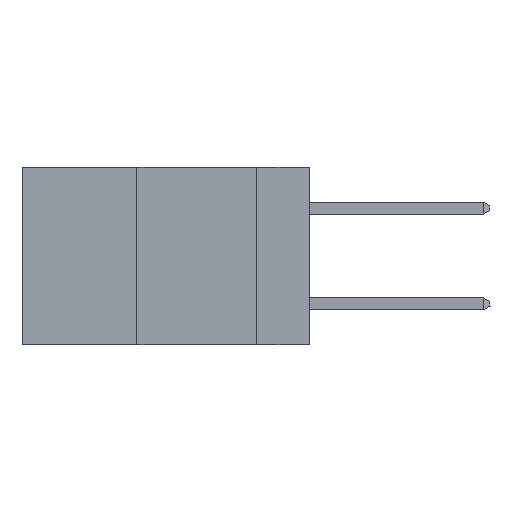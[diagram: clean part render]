
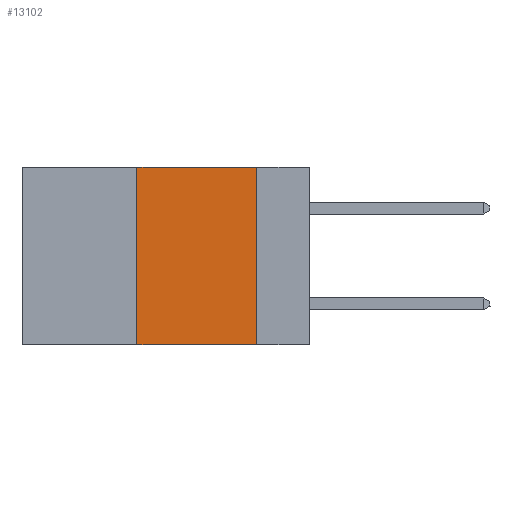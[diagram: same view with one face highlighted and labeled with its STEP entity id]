
A CAD part, left-side view. The second image highlights one B-rep face of the part: STEP entity #13102.
In plain terms, the highlighted planar face has unit normal (-1, 0, 0).
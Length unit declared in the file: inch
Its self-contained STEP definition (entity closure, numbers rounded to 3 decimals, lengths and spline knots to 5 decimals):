
#767 = ORIENTED_EDGE ( 'NONE', *, *, #16006, .F. ) ;
#4072 = ORIENTED_EDGE ( 'NONE', *, *, #23856, .F. ) ;
#5783 = CARTESIAN_POINT ( 'NONE',  ( 0., 0.11, -0.37 ) ) ;
#7121 = CARTESIAN_POINT ( 'NONE',  ( 0., 0.11, 0. ) ) ;
#8028 = VERTEX_POINT ( 'NONE', #39222 ) ;
#10230 = LINE ( 'NONE', #42570, #43635 ) ;
#11547 = DIRECTION ( 'NONE',  ( 0., -1., 0. ) ) ;
#12659 = CARTESIAN_POINT ( 'NONE',  ( 0., 0.6, 0. ) ) ;
#12852 = VECTOR ( 'NONE', #21249, 39.37008 ) ;
#13102 = ADVANCED_FACE ( 'NONE', ( #33027 ), #19463, .F. ) ;
#16006 = EDGE_CURVE ( 'NONE', #36220, #34450, #42230, .T. ) ;
#17598 = EDGE_CURVE ( 'NONE', #8028, #34450, #21129, .T. ) ;
#19024 = CARTESIAN_POINT ( 'NONE',  ( 0., 0.36, 0. ) ) ;
#19349 = CARTESIAN_POINT ( 'NONE',  ( 0., 0.6, -0.37 ) ) ;
#19463 = PLANE ( 'NONE',  #24217 ) ;
#21129 = LINE ( 'NONE', #19349, #30274 ) ;
#21249 = DIRECTION ( 'NONE',  ( 0., 0., 1. ) ) ;
#22064 = LINE ( 'NONE', #34894, #12852 ) ;
#22842 = DIRECTION ( 'NONE',  ( 0., -1., 0. ) ) ;
#23856 = EDGE_CURVE ( 'NONE', #8028, #38740, #22064, .T. ) ;
#23969 = VECTOR ( 'NONE', #34736, 39.37008 ) ;
#24217 = AXIS2_PLACEMENT_3D ( 'NONE', #12659, #36601, #36755 ) ;
#29252 = EDGE_CURVE ( 'NONE', #38740, #36220, #10230, .T. ) ;
#30274 = VECTOR ( 'NONE', #22842, 39.37008 ) ;
#30576 = ORIENTED_EDGE ( 'NONE', *, *, #29252, .F. ) ;
#31462 = EDGE_LOOP ( 'NONE', ( #767, #30576, #4072, #39186 ) ) ;
#33027 = FACE_OUTER_BOUND ( 'NONE', #31462, .T. ) ;
#34450 = VERTEX_POINT ( 'NONE', #5783 ) ;
#34736 = DIRECTION ( 'NONE',  ( 0., 0., -1. ) ) ;
#34894 = CARTESIAN_POINT ( 'NONE',  ( 0., 0.36, 0. ) ) ;
#36220 = VERTEX_POINT ( 'NONE', #42490 ) ;
#36601 = DIRECTION ( 'NONE',  ( 1., 0., 0. ) ) ;
#36755 = DIRECTION ( 'NONE',  ( 0., 0., -1. ) ) ;
#38740 = VERTEX_POINT ( 'NONE', #19024 ) ;
#39186 = ORIENTED_EDGE ( 'NONE', *, *, #17598, .T. ) ;
#39222 = CARTESIAN_POINT ( 'NONE',  ( 0., 0.36, -0.37 ) ) ;
#42230 = LINE ( 'NONE', #7121, #23969 ) ;
#42490 = CARTESIAN_POINT ( 'NONE',  ( 0., 0.11, 0. ) ) ;
#42570 = CARTESIAN_POINT ( 'NONE',  ( 0., 0.6, 0. ) ) ;
#43635 = VECTOR ( 'NONE', #11547, 39.37008 ) ;
